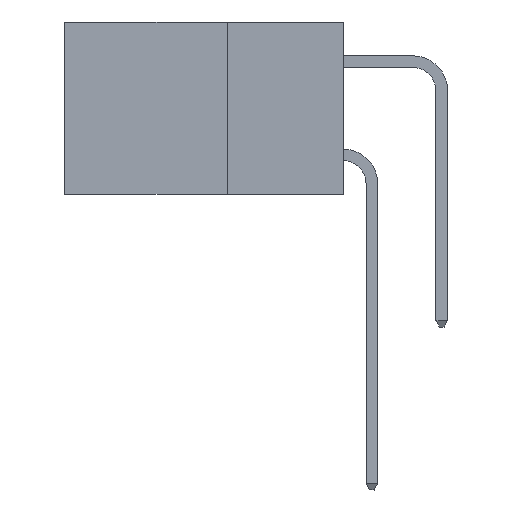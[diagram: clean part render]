
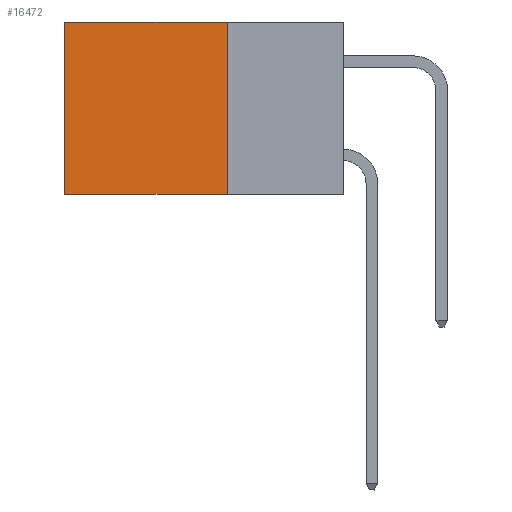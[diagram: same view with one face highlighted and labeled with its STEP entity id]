
A CAD part, left-side view. The second image highlights one B-rep face of the part: STEP entity #16472.
In plain terms, the highlighted planar face has unit normal (-1, 0, 0).
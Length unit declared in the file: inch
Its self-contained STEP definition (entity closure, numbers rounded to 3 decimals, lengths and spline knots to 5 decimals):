
#719 = CARTESIAN_POINT ( 'NONE',  ( 0.2615, 0.6, -0.37 ) ) ;
#802 = CARTESIAN_POINT ( 'NONE',  ( 0.2615, 0.25, -0.37 ) ) ;
#1186 = DIRECTION ( 'NONE',  ( 0., 1., 0. ) ) ;
#2341 = CARTESIAN_POINT ( 'NONE',  ( 0.2615, 0.25, 0. ) ) ;
#2947 = EDGE_CURVE ( 'NONE', #5286, #8346, #11122, .T. ) ;
#5045 = VERTEX_POINT ( 'NONE', #11233 ) ;
#5286 = VERTEX_POINT ( 'NONE', #2341 ) ;
#7060 = EDGE_LOOP ( 'NONE', ( #15152, #17234, #16043, #14016 ) ) ;
#7249 = PLANE ( 'NONE',  #8041 ) ;
#7330 = DIRECTION ( 'NONE',  ( 1., 0., 0. ) ) ;
#8041 = AXIS2_PLACEMENT_3D ( 'NONE', #12815, #7330, #10055 ) ;
#8346 = VERTEX_POINT ( 'NONE', #17766 ) ;
#8709 = FACE_OUTER_BOUND ( 'NONE', #7060, .T. ) ;
#9735 = CARTESIAN_POINT ( 'NONE',  ( 0.2615, 0.25, 0. ) ) ;
#10055 = DIRECTION ( 'NONE',  ( 0., 0., -1. ) ) ;
#10587 = EDGE_CURVE ( 'NONE', #5286, #14494, #17528, .T. ) ;
#11122 = LINE ( 'NONE', #9735, #13255 ) ;
#11233 = CARTESIAN_POINT ( 'NONE',  ( 0.2615, 0.6, -0.37 ) ) ;
#11446 = VECTOR ( 'NONE', #13350, 39.37008 ) ;
#11987 = DIRECTION ( 'NONE',  ( 0., 0., -1. ) ) ;
#12057 = CARTESIAN_POINT ( 'NONE',  ( 0.2615, 0.25, -0.37 ) ) ;
#12815 = CARTESIAN_POINT ( 'NONE',  ( 0.2615, 0.25, -0.37 ) ) ;
#13255 = VECTOR ( 'NONE', #15316, 39.37008 ) ;
#13350 = DIRECTION ( 'NONE',  ( 0., 0., -1. ) ) ;
#13476 = VECTOR ( 'NONE', #11987, 39.37008 ) ;
#13811 = CARTESIAN_POINT ( 'NONE',  ( 0.2615, 0.25, -0.37 ) ) ;
#13859 = EDGE_CURVE ( 'NONE', #8346, #5045, #14512, .T. ) ;
#14016 = ORIENTED_EDGE ( 'NONE', *, *, #2947, .T. ) ;
#14494 = VERTEX_POINT ( 'NONE', #12057 ) ;
#14512 = LINE ( 'NONE', #719, #11446 ) ;
#14759 = VECTOR ( 'NONE', #1186, 39.37008 ) ;
#15095 = LINE ( 'NONE', #13811, #14759 ) ;
#15152 = ORIENTED_EDGE ( 'NONE', *, *, #13859, .T. ) ;
#15316 = DIRECTION ( 'NONE',  ( 0., 1., 0. ) ) ;
#16043 = ORIENTED_EDGE ( 'NONE', *, *, #10587, .F. ) ;
#16472 = ADVANCED_FACE ( 'NONE', ( #8709 ), #7249, .F. ) ;
#17234 = ORIENTED_EDGE ( 'NONE', *, *, #17391, .F. ) ;
#17391 = EDGE_CURVE ( 'NONE', #14494, #5045, #15095, .T. ) ;
#17528 = LINE ( 'NONE', #802, #13476 ) ;
#17766 = CARTESIAN_POINT ( 'NONE',  ( 0.2615, 0.6, 0. ) ) ;
